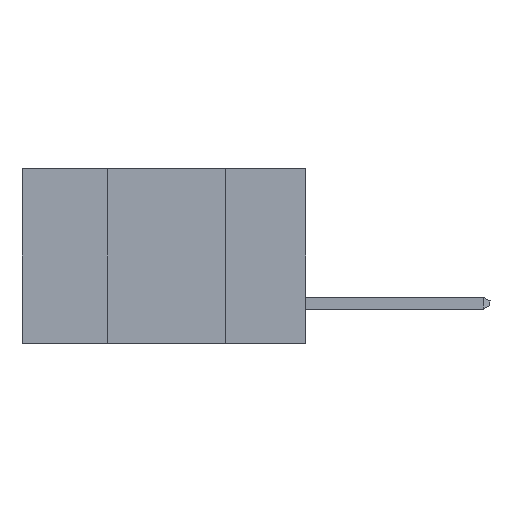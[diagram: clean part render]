
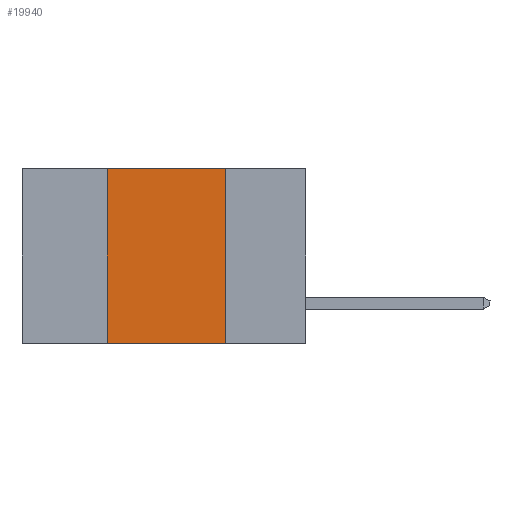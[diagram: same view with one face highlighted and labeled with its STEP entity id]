
A CAD part, left-side view. The second image highlights one B-rep face of the part: STEP entity #19940.
In plain terms, the highlighted planar face has unit normal (-1, 0, 0).
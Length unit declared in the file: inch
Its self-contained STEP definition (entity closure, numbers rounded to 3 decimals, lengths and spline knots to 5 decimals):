
#152 = DIRECTION ( 'NONE',  ( 0., 0., 1. ) ) ;
#317 = ORIENTED_EDGE ( 'NONE', *, *, #16156, .T. ) ;
#595 = VERTEX_POINT ( 'NONE', #8334 ) ;
#813 = VERTEX_POINT ( 'NONE', #2004 ) ;
#1116 = DIRECTION ( 'NONE',  ( 0., -1., 0. ) ) ;
#1809 = CARTESIAN_POINT ( 'NONE',  ( 0., 0.42, -0.37 ) ) ;
#2004 = CARTESIAN_POINT ( 'NONE',  ( 0., 0.17, -0.37 ) ) ;
#3302 = CARTESIAN_POINT ( 'NONE',  ( 0., 0.42, -0.37 ) ) ;
#3446 = CARTESIAN_POINT ( 'NONE',  ( 0., 0.6, -0.37 ) ) ;
#3705 = ORIENTED_EDGE ( 'NONE', *, *, #19544, .F. ) ;
#4501 = VECTOR ( 'NONE', #152, 39.37008 ) ;
#4911 = EDGE_LOOP ( 'NONE', ( #19721, #3705, #10432, #317 ) ) ;
#5271 = EDGE_CURVE ( 'NONE', #18366, #595, #18827, .T. ) ;
#5774 = EDGE_CURVE ( 'NONE', #18629, #813, #12726, .T. ) ;
#5787 = DIRECTION ( 'NONE',  ( 1., 0., 0. ) ) ;
#7986 = LINE ( 'NONE', #3446, #8714 ) ;
#8334 = CARTESIAN_POINT ( 'NONE',  ( 0., 0.42, 0. ) ) ;
#8714 = VECTOR ( 'NONE', #19070, 39.37008 ) ;
#8915 = LINE ( 'NONE', #10650, #19307 ) ;
#9634 = DIRECTION ( 'NONE',  ( 0., 0., -1. ) ) ;
#10432 = ORIENTED_EDGE ( 'NONE', *, *, #5271, .F. ) ;
#10650 = CARTESIAN_POINT ( 'NONE',  ( 0., 0.6, 0. ) ) ;
#12720 = VECTOR ( 'NONE', #9634, 39.37008 ) ;
#12726 = LINE ( 'NONE', #18987, #12720 ) ;
#13600 = FACE_OUTER_BOUND ( 'NONE', #4911, .T. ) ;
#13697 = CARTESIAN_POINT ( 'NONE',  ( 0., 0.6, 0. ) ) ;
#13893 = DIRECTION ( 'NONE',  ( 0., 0., -1. ) ) ;
#15803 = CARTESIAN_POINT ( 'NONE',  ( 0., 0.17, 0. ) ) ;
#16156 = EDGE_CURVE ( 'NONE', #18366, #813, #7986, .T. ) ;
#18229 = PLANE ( 'NONE',  #19602 ) ;
#18366 = VERTEX_POINT ( 'NONE', #3302 ) ;
#18629 = VERTEX_POINT ( 'NONE', #15803 ) ;
#18827 = LINE ( 'NONE', #1809, #4501 ) ;
#18987 = CARTESIAN_POINT ( 'NONE',  ( 0., 0.17, -0.37 ) ) ;
#19070 = DIRECTION ( 'NONE',  ( 0., -1., 0. ) ) ;
#19307 = VECTOR ( 'NONE', #1116, 39.37008 ) ;
#19544 = EDGE_CURVE ( 'NONE', #595, #18629, #8915, .T. ) ;
#19602 = AXIS2_PLACEMENT_3D ( 'NONE', #13697, #5787, #13893 ) ;
#19721 = ORIENTED_EDGE ( 'NONE', *, *, #5774, .F. ) ;
#19940 = ADVANCED_FACE ( 'NONE', ( #13600 ), #18229, .F. ) ;
